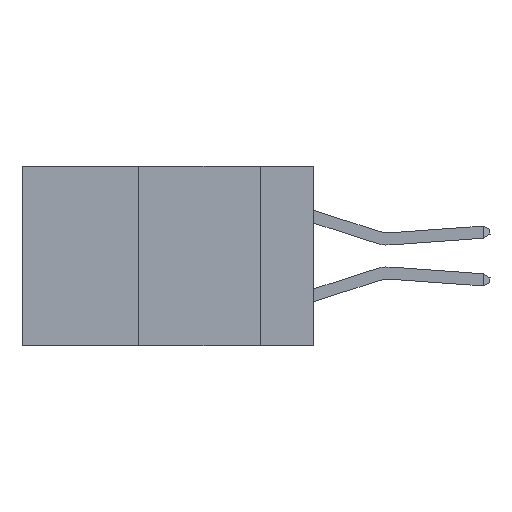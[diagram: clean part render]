
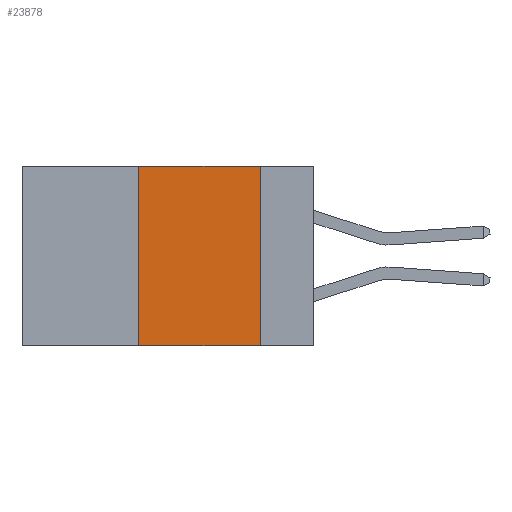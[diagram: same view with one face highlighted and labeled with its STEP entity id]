
A CAD part, left-side view. The second image highlights one B-rep face of the part: STEP entity #23878.
In plain terms, the highlighted planar face has unit normal (-1, 0, 0).
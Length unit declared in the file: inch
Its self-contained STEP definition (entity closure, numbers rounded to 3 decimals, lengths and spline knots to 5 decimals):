
#2435 = CARTESIAN_POINT ( 'NONE',  ( 0., 0.11, 0. ) ) ;
#3207 = CARTESIAN_POINT ( 'NONE',  ( 0., 0.36, 0. ) ) ;
#4351 = LINE ( 'NONE', #12609, #7500 ) ;
#5143 = VERTEX_POINT ( 'NONE', #18233 ) ;
#5784 = ORIENTED_EDGE ( 'NONE', *, *, #6364, .F. ) ;
#6224 = CARTESIAN_POINT ( 'NONE',  ( 0., 0.36, 0. ) ) ;
#6364 = EDGE_CURVE ( 'NONE', #36607, #24877, #33804, .T. ) ;
#7500 = VECTOR ( 'NONE', #12462, 39.37008 ) ;
#7530 = FACE_OUTER_BOUND ( 'NONE', #40451, .T. ) ;
#8204 = LINE ( 'NONE', #15175, #12441 ) ;
#12281 = LINE ( 'NONE', #3207, #33326 ) ;
#12441 = VECTOR ( 'NONE', #18532, 39.37008 ) ;
#12462 = DIRECTION ( 'NONE',  ( 0., -1., 0. ) ) ;
#12609 = CARTESIAN_POINT ( 'NONE',  ( 0., 0.6, -0.37 ) ) ;
#13345 = DIRECTION ( 'NONE',  ( 0., 0., 1. ) ) ;
#14964 = DIRECTION ( 'NONE',  ( 0., 0., -1. ) ) ;
#15175 = CARTESIAN_POINT ( 'NONE',  ( 0., 0.6, 0. ) ) ;
#15441 = ORIENTED_EDGE ( 'NONE', *, *, #16992, .F. ) ;
#15456 = AXIS2_PLACEMENT_3D ( 'NONE', #17894, #33904, #14964 ) ;
#16223 = CARTESIAN_POINT ( 'NONE',  ( 0., 0.11, -0.37 ) ) ;
#16992 = EDGE_CURVE ( 'NONE', #22957, #36607, #8204, .T. ) ;
#17894 = CARTESIAN_POINT ( 'NONE',  ( 0., 0.6, 0. ) ) ;
#18233 = CARTESIAN_POINT ( 'NONE',  ( 0., 0.36, -0.37 ) ) ;
#18532 = DIRECTION ( 'NONE',  ( 0., -1., 0. ) ) ;
#22957 = VERTEX_POINT ( 'NONE', #6224 ) ;
#23878 = ADVANCED_FACE ( 'NONE', ( #7530 ), #31258, .F. ) ;
#24877 = VERTEX_POINT ( 'NONE', #16223 ) ;
#29463 = DIRECTION ( 'NONE',  ( 0., 0., -1. ) ) ;
#31258 = PLANE ( 'NONE',  #15456 ) ;
#31294 = EDGE_CURVE ( 'NONE', #5143, #24877, #4351, .T. ) ;
#32252 = VECTOR ( 'NONE', #29463, 39.37008 ) ;
#33326 = VECTOR ( 'NONE', #13345, 39.37008 ) ;
#33354 = ORIENTED_EDGE ( 'NONE', *, *, #31294, .T. ) ;
#33804 = LINE ( 'NONE', #2435, #32252 ) ;
#33904 = DIRECTION ( 'NONE',  ( 1., 0., 0. ) ) ;
#34430 = CARTESIAN_POINT ( 'NONE',  ( 0., 0.11, 0. ) ) ;
#36607 = VERTEX_POINT ( 'NONE', #34430 ) ;
#38321 = ORIENTED_EDGE ( 'NONE', *, *, #43095, .F. ) ;
#40451 = EDGE_LOOP ( 'NONE', ( #5784, #15441, #38321, #33354 ) ) ;
#43095 = EDGE_CURVE ( 'NONE', #5143, #22957, #12281, .T. ) ;
